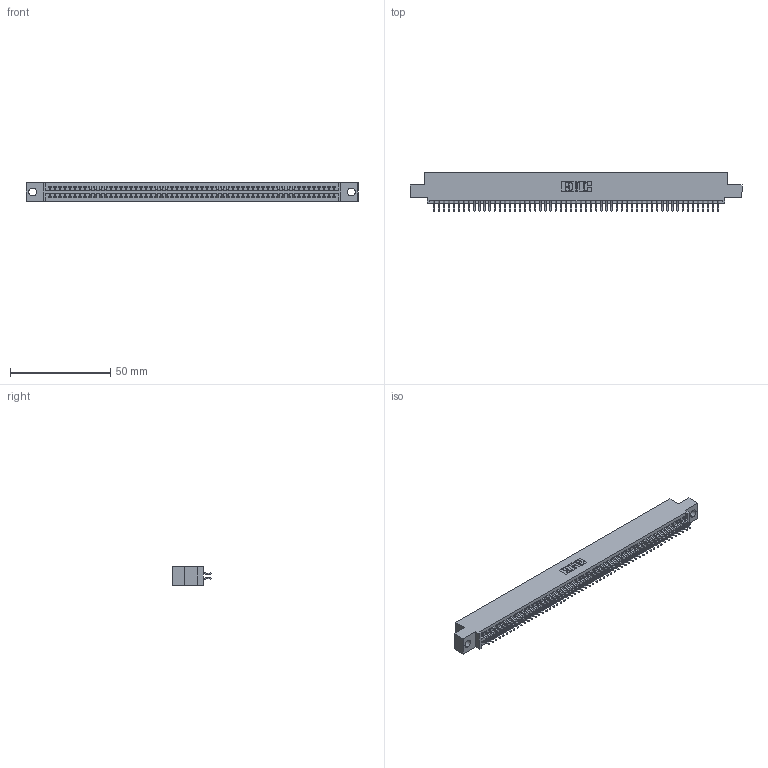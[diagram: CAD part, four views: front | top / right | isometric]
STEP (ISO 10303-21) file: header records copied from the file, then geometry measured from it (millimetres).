
FILE_DESCRIPTION (( 'STEP AP203' ), '1' );
FILE_NAME ('345-114-556-504.STEP', '2021-05-25T15:14:53', ( '' ), ( '' ), 'SwSTEP 2.0', 'SolidWorks 2020', '' );
FILE_SCHEMA (( 'CONFIG_CONTROL_DESIGN' ));
Length unit declared in the file: inch
Products named in the file (3): 345-292-001_556 Tail; 345 Part_0.110 Offset - 0.156 Dia-TI; 345-114-556-504
Assembly tree (115 placements, depth 2):
  345-114-556-504
    345 Part_0.110 Offset - 0.156 Dia-TI
    345-292-001_556 Tail  x114
Bounding box: 165.99 x 19.24 x 9.4 mm (x, y, z)
Volume: 16079.7 mm3; surface area: 23903.7 mm2
Topology: 115 solids, 115 shells, 6528 faces, 19427 edges, 12798 vertices
Faces by surface type: plane 4316, cylinder 2212
Entity records: 43475 total; most frequent: CARTESIAN_POINT 7294, ORIENTED_EDGE 7214, DIRECTION 6399, EDGE_CURVE 3607, LINE 3239, VECTOR 3239, VERTEX_POINT 2402, AXIS2_PLACEMENT_3D 1580
